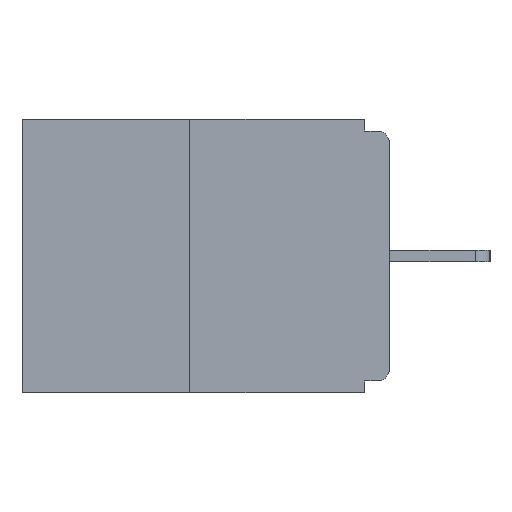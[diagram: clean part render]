
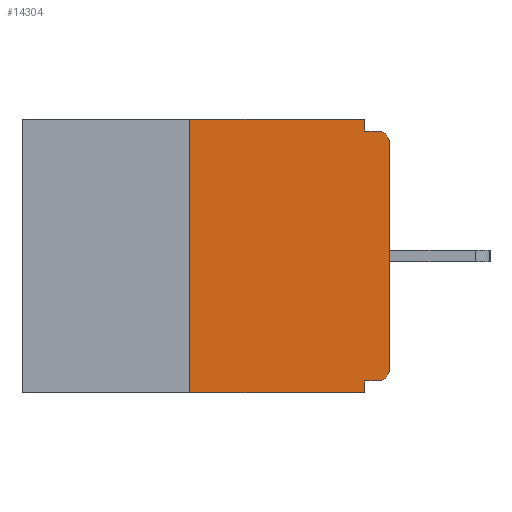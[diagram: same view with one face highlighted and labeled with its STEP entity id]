
A CAD part, left-side view. The second image highlights one B-rep face of the part: STEP entity #14304.
In plain terms, the highlighted planar face has unit normal (-1, 0, 0).
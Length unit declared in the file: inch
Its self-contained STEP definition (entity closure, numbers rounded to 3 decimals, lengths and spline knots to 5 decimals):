
#667 = CARTESIAN_POINT ( 'NONE',  ( 0., 0., -0.03 ) ) ;
#691 = LINE ( 'NONE', #14448, #15620 ) ;
#746 = CARTESIAN_POINT ( 'NONE',  ( 0., 0.015, -0.328 ) ) ;
#1196 = CARTESIAN_POINT ( 'NONE',  ( 0., 0.031, -0.015 ) ) ;
#1263 = AXIS2_PLACEMENT_3D ( 'NONE', #13534, #12121, #5587 ) ;
#1681 = LINE ( 'NONE', #3104, #14770 ) ;
#1975 = VERTEX_POINT ( 'NONE', #2487 ) ;
#2369 = VECTOR ( 'NONE', #3780, 39.37008 ) ;
#2487 = CARTESIAN_POINT ( 'NONE',  ( 0., 0.031, 0. ) ) ;
#2718 = EDGE_LOOP ( 'NONE', ( #5276, #7974, #15291, #15846, #16768, #16112, #12415, #10404, #3698, #10071 ) ) ;
#2944 = DIRECTION ( 'NONE',  ( 0., -1., 0. ) ) ;
#3086 = VERTEX_POINT ( 'NONE', #746 ) ;
#3104 = CARTESIAN_POINT ( 'NONE',  ( 0., 0.25, 0. ) ) ;
#3360 = EDGE_CURVE ( 'NONE', #13654, #13602, #1681, .T. ) ;
#3546 = CARTESIAN_POINT ( 'NONE',  ( 0., 0.25, 0. ) ) ;
#3582 = EDGE_CURVE ( 'NONE', #3086, #8454, #15719, .T. ) ;
#3698 = ORIENTED_EDGE ( 'NONE', *, *, #7879, .F. ) ;
#3780 = DIRECTION ( 'NONE',  ( 0., -1., 0. ) ) ;
#3998 = EDGE_CURVE ( 'NONE', #13654, #14154, #5105, .T. ) ;
#5105 = LINE ( 'NONE', #13069, #2369 ) ;
#5276 = ORIENTED_EDGE ( 'NONE', *, *, #9532, .F. ) ;
#5587 = DIRECTION ( 'NONE',  ( 0., 0., -1. ) ) ;
#6057 = VECTOR ( 'NONE', #10630, 39.37008 ) ;
#6252 = CARTESIAN_POINT ( 'NONE',  ( 0., 0.015, -0.015 ) ) ;
#6279 = DIRECTION ( 'NONE',  ( 0., 1., 0. ) ) ;
#6678 = VECTOR ( 'NONE', #6903, 39.37008 ) ;
#6747 = VERTEX_POINT ( 'NONE', #1196 ) ;
#6903 = DIRECTION ( 'NONE',  ( 0., 0., -1. ) ) ;
#7161 = VECTOR ( 'NONE', #2944, 39.37008 ) ;
#7512 = EDGE_CURVE ( 'NONE', #1975, #6747, #13436, .T. ) ;
#7718 = VECTOR ( 'NONE', #6279, 39.37008 ) ;
#7750 = CIRCLE ( 'NONE', #1263, 0.015 ) ;
#7863 = VERTEX_POINT ( 'NONE', #6252 ) ;
#7879 = EDGE_CURVE ( 'NONE', #6747, #7863, #9062, .T. ) ;
#7891 = CARTESIAN_POINT ( 'NONE',  ( 0., 0., 0. ) ) ;
#7974 = ORIENTED_EDGE ( 'NONE', *, *, #3360, .F. ) ;
#8205 = CARTESIAN_POINT ( 'NONE',  ( 0., 0.031, 0. ) ) ;
#8454 = VERTEX_POINT ( 'NONE', #17447 ) ;
#8701 = DIRECTION ( 'NONE',  ( 0., 0., -1. ) ) ;
#9004 = CARTESIAN_POINT ( 'NONE',  ( 0., 0., -0.328 ) ) ;
#9062 = LINE ( 'NONE', #14371, #16118 ) ;
#9080 = CARTESIAN_POINT ( 'NONE',  ( 0., 0., -0.313 ) ) ;
#9272 = EDGE_CURVE ( 'NONE', #3086, #11285, #15306, .T. ) ;
#9532 = EDGE_CURVE ( 'NONE', #13602, #1975, #16351, .T. ) ;
#9734 = DIRECTION ( 'NONE',  ( 0., 0., 1. ) ) ;
#10071 = ORIENTED_EDGE ( 'NONE', *, *, #7512, .F. ) ;
#10234 = EDGE_CURVE ( 'NONE', #8454, #14154, #691, .T. ) ;
#10404 = ORIENTED_EDGE ( 'NONE', *, *, #12328, .T. ) ;
#10445 = VERTEX_POINT ( 'NONE', #667 ) ;
#10630 = DIRECTION ( 'NONE',  ( 0., 0., 1. ) ) ;
#10642 = CARTESIAN_POINT ( 'NONE',  ( 0., 0.031, -0.343 ) ) ;
#10690 = EDGE_CURVE ( 'NONE', #11285, #10445, #14611, .T. ) ;
#11256 = DIRECTION ( 'NONE',  ( 0., 0., -1. ) ) ;
#11285 = VERTEX_POINT ( 'NONE', #9080 ) ;
#12074 = DIRECTION ( 'NONE',  ( 0., 0., -1. ) ) ;
#12121 = DIRECTION ( 'NONE',  ( -1., 0., 0. ) ) ;
#12328 = EDGE_CURVE ( 'NONE', #10445, #7863, #7750, .T. ) ;
#12415 = ORIENTED_EDGE ( 'NONE', *, *, #10690, .T. ) ;
#12730 = AXIS2_PLACEMENT_3D ( 'NONE', #17139, #14078, #8701 ) ;
#12863 = FACE_OUTER_BOUND ( 'NONE', #2718, .T. ) ;
#13059 = DIRECTION ( 'NONE',  ( 0., -1., 0. ) ) ;
#13069 = CARTESIAN_POINT ( 'NONE',  ( 0., 0.46, -0.343 ) ) ;
#13436 = LINE ( 'NONE', #8205, #6678 ) ;
#13534 = CARTESIAN_POINT ( 'NONE',  ( 0., 0.015, -0.03 ) ) ;
#13602 = VERTEX_POINT ( 'NONE', #3546 ) ;
#13654 = VERTEX_POINT ( 'NONE', #17295 ) ;
#14078 = DIRECTION ( 'NONE',  ( 1., 0., 0. ) ) ;
#14154 = VERTEX_POINT ( 'NONE', #10642 ) ;
#14304 = ADVANCED_FACE ( 'NONE', ( #12863 ), #14342, .F. ) ;
#14342 = PLANE ( 'NONE',  #12730 ) ;
#14371 = CARTESIAN_POINT ( 'NONE',  ( 0., 0., -0.015 ) ) ;
#14448 = CARTESIAN_POINT ( 'NONE',  ( 0., 0.031, -0.343 ) ) ;
#14611 = LINE ( 'NONE', #7891, #6057 ) ;
#14770 = VECTOR ( 'NONE', #9734, 39.37008 ) ;
#14868 = CARTESIAN_POINT ( 'NONE',  ( 0., 0.46, 0. ) ) ;
#15291 = ORIENTED_EDGE ( 'NONE', *, *, #3998, .T. ) ;
#15306 = CIRCLE ( 'NONE', #15592, 0.015 ) ;
#15319 = DIRECTION ( 'NONE',  ( -1., 0., 0. ) ) ;
#15490 = CARTESIAN_POINT ( 'NONE',  ( 0., 0.015, -0.313 ) ) ;
#15592 = AXIS2_PLACEMENT_3D ( 'NONE', #15490, #15319, #11256 ) ;
#15620 = VECTOR ( 'NONE', #12074, 39.37008 ) ;
#15719 = LINE ( 'NONE', #9004, #7718 ) ;
#15846 = ORIENTED_EDGE ( 'NONE', *, *, #10234, .F. ) ;
#16112 = ORIENTED_EDGE ( 'NONE', *, *, #9272, .T. ) ;
#16118 = VECTOR ( 'NONE', #13059, 39.37008 ) ;
#16351 = LINE ( 'NONE', #14868, #7161 ) ;
#16768 = ORIENTED_EDGE ( 'NONE', *, *, #3582, .F. ) ;
#17139 = CARTESIAN_POINT ( 'NONE',  ( 0., 0.46, 0. ) ) ;
#17295 = CARTESIAN_POINT ( 'NONE',  ( 0., 0.25, -0.343 ) ) ;
#17447 = CARTESIAN_POINT ( 'NONE',  ( 0., 0.031, -0.328 ) ) ;
